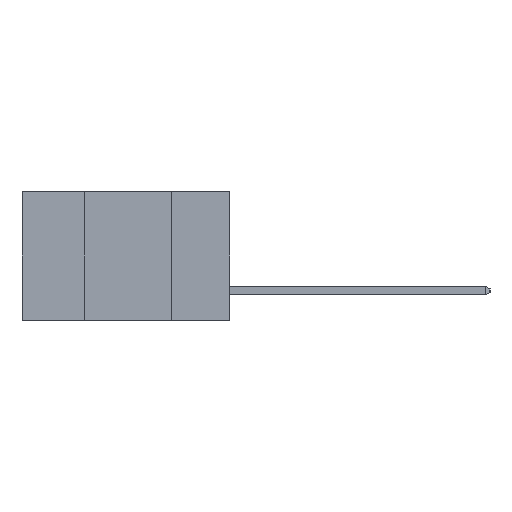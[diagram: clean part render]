
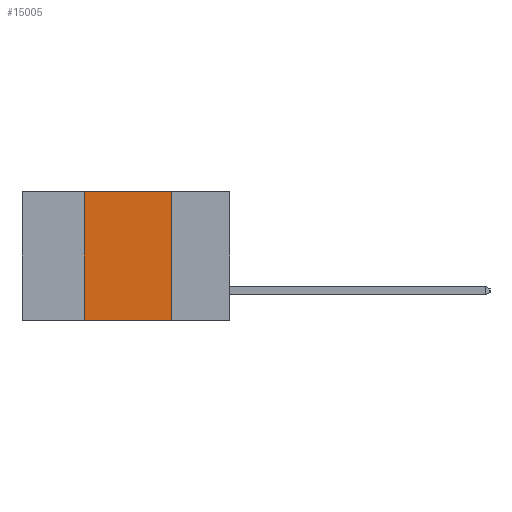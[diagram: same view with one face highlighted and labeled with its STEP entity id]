
A CAD part, left-side view. The second image highlights one B-rep face of the part: STEP entity #15005.
In plain terms, the highlighted planar face has unit normal (-1, 0, 0).
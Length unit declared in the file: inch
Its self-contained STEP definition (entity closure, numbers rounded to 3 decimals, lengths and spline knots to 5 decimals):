
#175 = DIRECTION ( 'NONE',  ( 0., 0., -1. ) ) ;
#202 = DIRECTION ( 'NONE',  ( 0., -1., 0. ) ) ;
#468 = LINE ( 'NONE', #2542, #5039 ) ;
#765 = CARTESIAN_POINT ( 'NONE',  ( 0., 0.17, -0.37 ) ) ;
#802 = ORIENTED_EDGE ( 'NONE', *, *, #1736, .F. ) ;
#1736 = EDGE_CURVE ( 'NONE', #8025, #24656, #3587, .T. ) ;
#2360 = VECTOR ( 'NONE', #175, 39.37008 ) ;
#2542 = CARTESIAN_POINT ( 'NONE',  ( 0., 0.42, -0.37 ) ) ;
#3587 = LINE ( 'NONE', #765, #2360 ) ;
#3988 = ORIENTED_EDGE ( 'NONE', *, *, #17538, .F. ) ;
#4435 = CARTESIAN_POINT ( 'NONE',  ( 0., 0.17, 0. ) ) ;
#4453 = FACE_OUTER_BOUND ( 'NONE', #16836, .T. ) ;
#4502 = DIRECTION ( 'NONE',  ( 0., 0., 1. ) ) ;
#5039 = VECTOR ( 'NONE', #4502, 39.37008 ) ;
#6683 = VECTOR ( 'NONE', #202, 39.37008 ) ;
#7290 = EDGE_CURVE ( 'NONE', #21653, #24656, #7907, .T. ) ;
#7415 = LINE ( 'NONE', #22142, #17161 ) ;
#7907 = LINE ( 'NONE', #23484, #6683 ) ;
#7918 = ORIENTED_EDGE ( 'NONE', *, *, #18274, .F. ) ;
#8025 = VERTEX_POINT ( 'NONE', #4435 ) ;
#8260 = PLANE ( 'NONE',  #16707 ) ;
#9243 = VERTEX_POINT ( 'NONE', #16094 ) ;
#10210 = DIRECTION ( 'NONE',  ( 1., 0., 0. ) ) ;
#12541 = DIRECTION ( 'NONE',  ( 0., -1., 0. ) ) ;
#13017 = CARTESIAN_POINT ( 'NONE',  ( 0., 0.42, -0.37 ) ) ;
#15005 = ADVANCED_FACE ( 'NONE', ( #4453 ), #8260, .F. ) ;
#16094 = CARTESIAN_POINT ( 'NONE',  ( 0., 0.42, 0. ) ) ;
#16707 = AXIS2_PLACEMENT_3D ( 'NONE', #19863, #10210, #23738 ) ;
#16836 = EDGE_LOOP ( 'NONE', ( #802, #7918, #3988, #18396 ) ) ;
#17161 = VECTOR ( 'NONE', #12541, 39.37008 ) ;
#17538 = EDGE_CURVE ( 'NONE', #21653, #9243, #468, .T. ) ;
#18274 = EDGE_CURVE ( 'NONE', #9243, #8025, #7415, .T. ) ;
#18396 = ORIENTED_EDGE ( 'NONE', *, *, #7290, .T. ) ;
#19863 = CARTESIAN_POINT ( 'NONE',  ( 0., 0.6, 0. ) ) ;
#20671 = CARTESIAN_POINT ( 'NONE',  ( 0., 0.17, -0.37 ) ) ;
#21653 = VERTEX_POINT ( 'NONE', #13017 ) ;
#22142 = CARTESIAN_POINT ( 'NONE',  ( 0., 0.6, 0. ) ) ;
#23484 = CARTESIAN_POINT ( 'NONE',  ( 0., 0.6, -0.37 ) ) ;
#23738 = DIRECTION ( 'NONE',  ( 0., 0., -1. ) ) ;
#24656 = VERTEX_POINT ( 'NONE', #20671 ) ;
